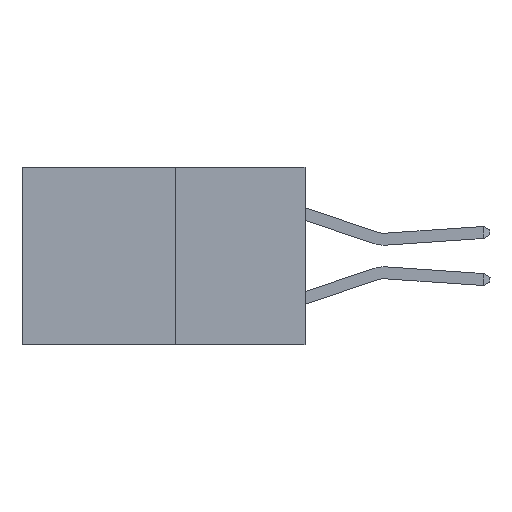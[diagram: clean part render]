
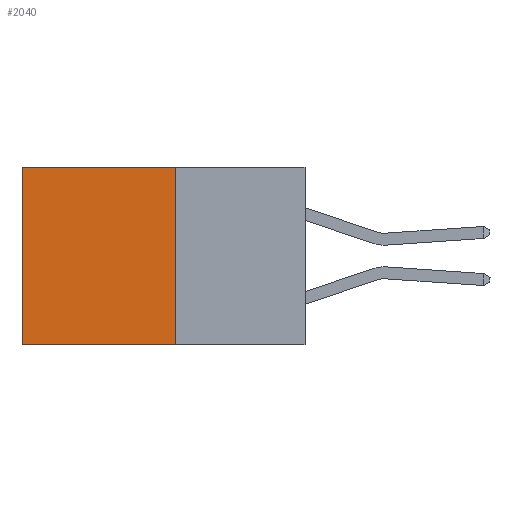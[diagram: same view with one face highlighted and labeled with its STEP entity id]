
A CAD part, left-side view. The second image highlights one B-rep face of the part: STEP entity #2040.
In plain terms, the highlighted planar face has unit normal (-1, 0, 0).
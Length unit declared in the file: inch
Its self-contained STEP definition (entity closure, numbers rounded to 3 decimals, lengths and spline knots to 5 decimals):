
#1613 = VECTOR ( 'NONE', #24608, 39.37008 ) ;
#1866 = LINE ( 'NONE', #11832, #9571 ) ;
#2040 = ADVANCED_FACE ( 'NONE', ( #19070 ), #17120, .F. ) ;
#2419 = LINE ( 'NONE', #21129, #1613 ) ;
#3709 = ORIENTED_EDGE ( 'NONE', *, *, #3772, .T. ) ;
#3772 = EDGE_CURVE ( 'NONE', #24389, #33162, #2419, .T. ) ;
#3989 = CARTESIAN_POINT ( 'NONE',  ( 0.277, 0.59, -0.37 ) ) ;
#4540 = CARTESIAN_POINT ( 'NONE',  ( 0.277, 0.27, 0. ) ) ;
#5848 = VECTOR ( 'NONE', #13739, 39.37008 ) ;
#8793 = EDGE_CURVE ( 'NONE', #24389, #15552, #12714, .T. ) ;
#9571 = VECTOR ( 'NONE', #29684, 39.37008 ) ;
#11433 = CARTESIAN_POINT ( 'NONE',  ( 0.277, 0.59, -0.37 ) ) ;
#11832 = CARTESIAN_POINT ( 'NONE',  ( 0.277, 0.27, -0.37 ) ) ;
#12714 = LINE ( 'NONE', #13891, #5848 ) ;
#12887 = EDGE_CURVE ( 'NONE', #15552, #21342, #1866, .T. ) ;
#13739 = DIRECTION ( 'NONE',  ( 0., 0., -1. ) ) ;
#13891 = CARTESIAN_POINT ( 'NONE',  ( 0.277, 0.27, -0.37 ) ) ;
#15552 = VERTEX_POINT ( 'NONE', #31312 ) ;
#16085 = ORIENTED_EDGE ( 'NONE', *, *, #8793, .F. ) ;
#16744 = DIRECTION ( 'NONE',  ( 0., 0., -1. ) ) ;
#17120 = PLANE ( 'NONE',  #27620 ) ;
#17147 = DIRECTION ( 'NONE',  ( 1., 0., 0. ) ) ;
#17725 = CARTESIAN_POINT ( 'NONE',  ( 0.277, 0.27, -0.37 ) ) ;
#18552 = CARTESIAN_POINT ( 'NONE',  ( 0.277, 0.59, 0. ) ) ;
#19070 = FACE_OUTER_BOUND ( 'NONE', #25233, .T. ) ;
#21129 = CARTESIAN_POINT ( 'NONE',  ( 0.277, 0.27, 0. ) ) ;
#21342 = VERTEX_POINT ( 'NONE', #11433 ) ;
#22014 = DIRECTION ( 'NONE',  ( 0., 0., -1. ) ) ;
#24251 = EDGE_CURVE ( 'NONE', #33162, #21342, #29436, .T. ) ;
#24389 = VERTEX_POINT ( 'NONE', #4540 ) ;
#24608 = DIRECTION ( 'NONE',  ( 0., 1., 0. ) ) ;
#24671 = ORIENTED_EDGE ( 'NONE', *, *, #12887, .F. ) ;
#25233 = EDGE_LOOP ( 'NONE', ( #29802, #24671, #16085, #3709 ) ) ;
#27620 = AXIS2_PLACEMENT_3D ( 'NONE', #17725, #17147, #16744 ) ;
#28640 = VECTOR ( 'NONE', #22014, 39.37008 ) ;
#29436 = LINE ( 'NONE', #3989, #28640 ) ;
#29684 = DIRECTION ( 'NONE',  ( 0., 1., 0. ) ) ;
#29802 = ORIENTED_EDGE ( 'NONE', *, *, #24251, .T. ) ;
#31312 = CARTESIAN_POINT ( 'NONE',  ( 0.277, 0.27, -0.37 ) ) ;
#33162 = VERTEX_POINT ( 'NONE', #18552 ) ;
